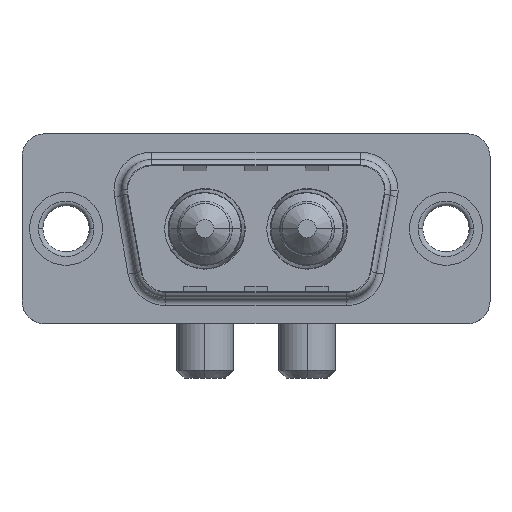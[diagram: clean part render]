
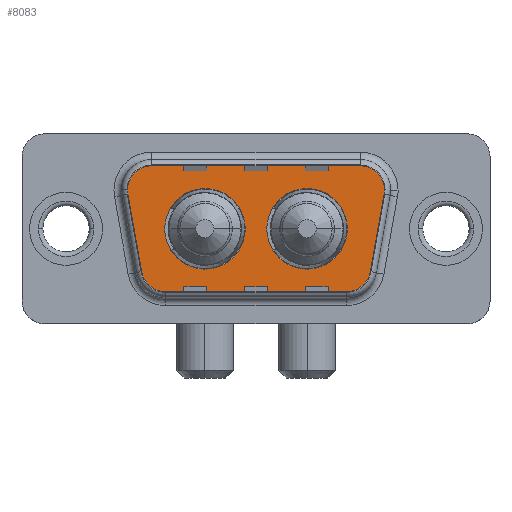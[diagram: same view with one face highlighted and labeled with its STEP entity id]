
A CAD part, top view. The second image highlights one B-rep face of the part: STEP entity #8083.
In plain terms, the highlighted planar face has unit normal (0, 0, 1).
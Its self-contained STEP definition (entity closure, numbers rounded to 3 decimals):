
#75 = ORIENTED_EDGE ( 'NONE', *, *, #1168, .F. ) ;
#261 = VECTOR ( 'NONE', #2243, 1000. ) ;
#572 = ORIENTED_EDGE ( 'NONE', *, *, #9629, .F. ) ;
#622 = CARTESIAN_POINT ( 'NONE',  ( 6.49, 0., 0. ) ) ;
#648 = CARTESIAN_POINT ( 'NONE',  ( 18.541, -4.9, 0. ) ) ;
#673 = EDGE_CURVE ( 'NONE', #2256, #5386, #6381, .T. ) ;
#731 = CARTESIAN_POINT ( 'NONE',  ( 6.459, -4.9, 0. ) ) ;
#738 = EDGE_CURVE ( 'NONE', #7917, #8794, #8589, .T. ) ;
#758 = LINE ( 'NONE', #1458, #261 ) ;
#880 = DIRECTION ( 'NONE',  ( 0.174, 0.985, 0. ) ) ;
#932 = LINE ( 'NONE', #3940, #2816 ) ;
#951 = CIRCLE ( 'NONE', #8822, 2. ) ;
#954 = DIRECTION ( 'NONE',  ( 1., 0., 0. ) ) ;
#1168 = EDGE_CURVE ( 'NONE', #5386, #2256, #3408, .T. ) ;
#1366 = EDGE_LOOP ( 'NONE', ( #75, #1653 ) ) ;
#1458 = CARTESIAN_POINT ( 'NONE',  ( 3.466, 2.553, 0. ) ) ;
#1478 = DIRECTION ( 'NONE',  ( 1., 0., 0. ) ) ;
#1617 = CARTESIAN_POINT ( 'NONE',  ( 21.534, 2.553, 0. ) ) ;
#1653 = ORIENTED_EDGE ( 'NONE', *, *, #673, .F. ) ;
#1710 = CARTESIAN_POINT ( 'NONE',  ( 5.436, 4.9, 0. ) ) ;
#1720 = AXIS2_PLACEMENT_3D ( 'NONE', #2742, #2647, #7236 ) ;
#1751 = DIRECTION ( 'NONE',  ( 1., 0., 0. ) ) ;
#1797 = EDGE_CURVE ( 'NONE', #6726, #5055, #758, .T. ) ;
#2036 = CARTESIAN_POINT ( 'NONE',  ( 19.564, 2.9, 0. ) ) ;
#2113 = CARTESIAN_POINT ( 'NONE',  ( 6.459, -2.9, 0. ) ) ;
#2233 = DIRECTION ( 'NONE',  ( 0., 0., 1. ) ) ;
#2243 = DIRECTION ( 'NONE',  ( 0.174, -0.985, 0. ) ) ;
#2256 = VERTEX_POINT ( 'NONE', #6564 ) ;
#2426 = CARTESIAN_POINT ( 'NONE',  ( 9.14, 0., 0. ) ) ;
#2492 = AXIS2_PLACEMENT_3D ( 'NONE', #2036, #6457, #2673 ) ;
#2499 = CIRCLE ( 'NONE', #7234, 2.65 ) ;
#2515 = AXIS2_PLACEMENT_3D ( 'NONE', #7080, #5482, #1751 ) ;
#2524 = CARTESIAN_POINT ( 'NONE',  ( 5.436, 4.9, 0. ) ) ;
#2647 = DIRECTION ( 'NONE',  ( 0., 0., 1. ) ) ;
#2673 = DIRECTION ( 'NONE',  ( -1., 0., 0. ) ) ;
#2742 = CARTESIAN_POINT ( 'NONE',  ( 5.436, 2.9, 0. ) ) ;
#2816 = VECTOR ( 'NONE', #3198, 1000. ) ;
#2841 = EDGE_CURVE ( 'NONE', #7685, #7711, #5943, .T. ) ;
#2882 = CARTESIAN_POINT ( 'NONE',  ( 4.489, -3.247, 0. ) ) ;
#2915 = DIRECTION ( 'NONE',  ( -1., 0., 0. ) ) ;
#2936 = VERTEX_POINT ( 'NONE', #648 ) ;
#2961 = FACE_BOUND ( 'NONE', #1366, .T. ) ;
#3010 = ORIENTED_EDGE ( 'NONE', *, *, #4777, .F. ) ;
#3015 = ORIENTED_EDGE ( 'NONE', *, *, #3679, .T. ) ;
#3110 = FACE_OUTER_BOUND ( 'NONE', #3134, .T. ) ;
#3134 = EDGE_LOOP ( 'NONE', ( #8499, #5524, #7908, #5784, #3560, #3015, #9502, #8425, #8173 ) ) ;
#3198 = DIRECTION ( 'NONE',  ( 1., 0., 0. ) ) ;
#3275 = CARTESIAN_POINT ( 'NONE',  ( 15.86, 0., 0. ) ) ;
#3408 = CIRCLE ( 'NONE', #4661, 2.65 ) ;
#3559 = CARTESIAN_POINT ( 'NONE',  ( 18.51, 0., 0. ) ) ;
#3560 = ORIENTED_EDGE ( 'NONE', *, *, #738, .T. ) ;
#3578 = VERTEX_POINT ( 'NONE', #6138 ) ;
#3587 = EDGE_CURVE ( 'NONE', #6800, #2936, #932, .T. ) ;
#3679 = EDGE_CURVE ( 'NONE', #8794, #6726, #5327, .T. ) ;
#3855 = CARTESIAN_POINT ( 'NONE',  ( 21.534, 2.553, 0. ) ) ;
#3940 = CARTESIAN_POINT ( 'NONE',  ( 6.459, -4.9, 0. ) ) ;
#4102 = DIRECTION ( 'NONE',  ( 0., 0., 1. ) ) ;
#4138 = EDGE_CURVE ( 'NONE', #2936, #3578, #4252, .T. ) ;
#4252 = CIRCLE ( 'NONE', #2515, 2. ) ;
#4375 = DIRECTION ( 'NONE',  ( -1., 0., 0. ) ) ;
#4528 = CARTESIAN_POINT ( 'NONE',  ( 18.541, -2.9, 0. ) ) ;
#4641 = DIRECTION ( 'NONE',  ( 0., 0., 1. ) ) ;
#4661 = AXIS2_PLACEMENT_3D ( 'NONE', #9278, #4102, #9326 ) ;
#4777 = EDGE_CURVE ( 'NONE', #7145, #7212, #2499, .T. ) ;
#5055 = VERTEX_POINT ( 'NONE', #2882 ) ;
#5259 = DIRECTION ( 'NONE',  ( 1., 0., 0. ) ) ;
#5327 = CIRCLE ( 'NONE', #1720, 2. ) ;
#5356 = CARTESIAN_POINT ( 'NONE',  ( 9.14, 0., 0. ) ) ;
#5374 = CARTESIAN_POINT ( 'NONE',  ( 21.564, 2.9, 0. ) ) ;
#5386 = VERTEX_POINT ( 'NONE', #3559 ) ;
#5418 = DIRECTION ( 'NONE',  ( 0., 0., 1. ) ) ;
#5482 = DIRECTION ( 'NONE',  ( 0., 0., 1. ) ) ;
#5521 = DIRECTION ( 'NONE',  ( 1., 0., 0. ) ) ;
#5524 = ORIENTED_EDGE ( 'NONE', *, *, #9537, .T. ) ;
#5640 = EDGE_CURVE ( 'NONE', #7711, #7917, #951, .T. ) ;
#5784 = ORIENTED_EDGE ( 'NONE', *, *, #5640, .T. ) ;
#5905 = PLANE ( 'NONE',  #7359 ) ;
#5943 = CIRCLE ( 'NONE', #2492, 2. ) ;
#5961 = CARTESIAN_POINT ( 'NONE',  ( 19.564, 2.9, 0. ) ) ;
#6074 = VECTOR ( 'NONE', #880, 1000. ) ;
#6127 = CARTESIAN_POINT ( 'NONE',  ( 11.79, 0., 0. ) ) ;
#6138 = CARTESIAN_POINT ( 'NONE',  ( 20.511, -3.247, 0. ) ) ;
#6140 = LINE ( 'NONE', #1617, #6074 ) ;
#6381 = CIRCLE ( 'NONE', #9549, 2.65 ) ;
#6457 = DIRECTION ( 'NONE',  ( 0., 0., 1. ) ) ;
#6482 = CIRCLE ( 'NONE', #9335, 2. ) ;
#6503 = EDGE_CURVE ( 'NONE', #5055, #6800, #6482, .T. ) ;
#6564 = CARTESIAN_POINT ( 'NONE',  ( 13.21, 0., 0. ) ) ;
#6659 = EDGE_LOOP ( 'NONE', ( #572, #3010 ) ) ;
#6726 = VERTEX_POINT ( 'NONE', #8082 ) ;
#6742 = DIRECTION ( 'NONE',  ( 0., 0., 1. ) ) ;
#6800 = VERTEX_POINT ( 'NONE', #731 ) ;
#7080 = CARTESIAN_POINT ( 'NONE',  ( 18.541, -2.9, 0. ) ) ;
#7145 = VERTEX_POINT ( 'NONE', #622 ) ;
#7212 = VERTEX_POINT ( 'NONE', #6127 ) ;
#7234 = AXIS2_PLACEMENT_3D ( 'NONE', #2426, #5418, #954 ) ;
#7236 = DIRECTION ( 'NONE',  ( 1., 0., 0. ) ) ;
#7359 = AXIS2_PLACEMENT_3D ( 'NONE', #4528, #8193, #5259 ) ;
#7685 = VERTEX_POINT ( 'NONE', #3855 ) ;
#7711 = VERTEX_POINT ( 'NONE', #5374 ) ;
#7821 = CIRCLE ( 'NONE', #9090, 2.65 ) ;
#7899 = DIRECTION ( 'NONE',  ( -1., 0., 0. ) ) ;
#7908 = ORIENTED_EDGE ( 'NONE', *, *, #2841, .T. ) ;
#7917 = VERTEX_POINT ( 'NONE', #9524 ) ;
#8082 = CARTESIAN_POINT ( 'NONE',  ( 3.466, 2.553, 0. ) ) ;
#8083 = ADVANCED_FACE ( 'NONE', ( #2961, #9673, #3110 ), #5905, .T. ) ;
#8173 = ORIENTED_EDGE ( 'NONE', *, *, #3587, .T. ) ;
#8193 = DIRECTION ( 'NONE',  ( 0., 0., 1. ) ) ;
#8425 = ORIENTED_EDGE ( 'NONE', *, *, #6503, .T. ) ;
#8499 = ORIENTED_EDGE ( 'NONE', *, *, #4138, .T. ) ;
#8589 = LINE ( 'NONE', #2524, #8758 ) ;
#8758 = VECTOR ( 'NONE', #7899, 1000. ) ;
#8794 = VERTEX_POINT ( 'NONE', #1710 ) ;
#8822 = AXIS2_PLACEMENT_3D ( 'NONE', #5961, #2233, #2915 ) ;
#9090 = AXIS2_PLACEMENT_3D ( 'NONE', #5356, #6742, #1478 ) ;
#9278 = CARTESIAN_POINT ( 'NONE',  ( 15.86, 0., 0. ) ) ;
#9326 = DIRECTION ( 'NONE',  ( 1., 0., 0. ) ) ;
#9335 = AXIS2_PLACEMENT_3D ( 'NONE', #2113, #9612, #4375 ) ;
#9502 = ORIENTED_EDGE ( 'NONE', *, *, #1797, .T. ) ;
#9524 = CARTESIAN_POINT ( 'NONE',  ( 19.564, 4.9, 0. ) ) ;
#9537 = EDGE_CURVE ( 'NONE', #3578, #7685, #6140, .T. ) ;
#9549 = AXIS2_PLACEMENT_3D ( 'NONE', #3275, #4641, #5521 ) ;
#9612 = DIRECTION ( 'NONE',  ( 0., 0., 1. ) ) ;
#9629 = EDGE_CURVE ( 'NONE', #7212, #7145, #7821, .T. ) ;
#9673 = FACE_BOUND ( 'NONE', #6659, .T. ) ;
